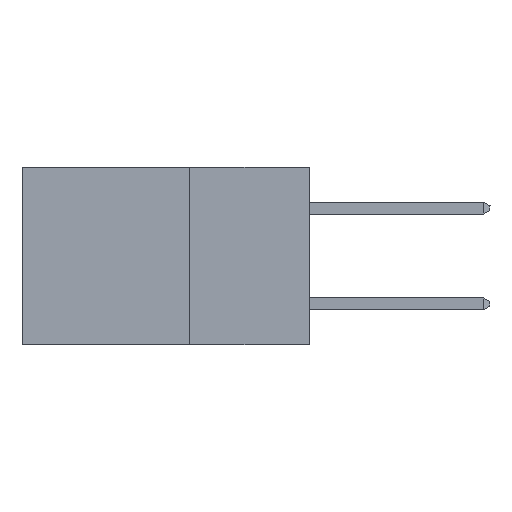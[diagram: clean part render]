
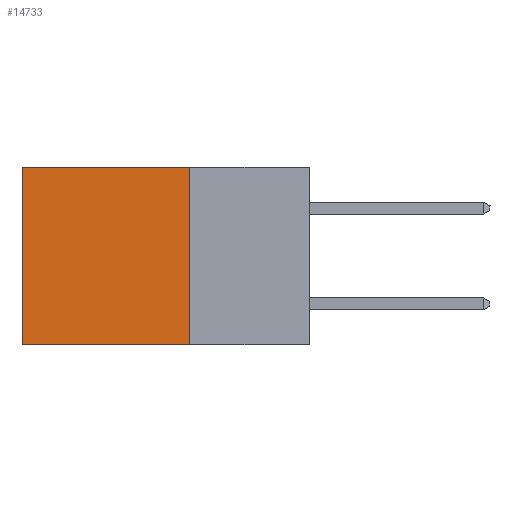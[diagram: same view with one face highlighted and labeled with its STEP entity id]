
A CAD part, left-side view. The second image highlights one B-rep face of the part: STEP entity #14733.
In plain terms, the highlighted planar face has unit normal (-1, 0, 0).
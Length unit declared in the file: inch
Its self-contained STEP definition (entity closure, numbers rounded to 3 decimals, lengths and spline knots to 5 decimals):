
#178 = VERTEX_POINT ( 'NONE', #4633 ) ;
#904 = LINE ( 'NONE', #6869, #1412 ) ;
#1408 = EDGE_CURVE ( 'NONE', #18609, #15009, #6712, .T. ) ;
#1412 = VECTOR ( 'NONE', #19752, 39.37008 ) ;
#1736 = CARTESIAN_POINT ( 'NONE',  ( 0.2875, 0.25, 0. ) ) ;
#2246 = CARTESIAN_POINT ( 'NONE',  ( 0.2875, 0.25, 0. ) ) ;
#3978 = AXIS2_PLACEMENT_3D ( 'NONE', #2246, #10109, #10245 ) ;
#4448 = ORIENTED_EDGE ( 'NONE', *, *, #20203, .F. ) ;
#4633 = CARTESIAN_POINT ( 'NONE',  ( 0.2875, 0.6, -0.37 ) ) ;
#5045 = LINE ( 'NONE', #8827, #16134 ) ;
#6611 = EDGE_LOOP ( 'NONE', ( #20382, #4448, #14657, #16684 ) ) ;
#6712 = LINE ( 'NONE', #8810, #16076 ) ;
#6869 = CARTESIAN_POINT ( 'NONE',  ( 0.2875, 0.6, 0. ) ) ;
#7322 = DIRECTION ( 'NONE',  ( 0., 1., 0. ) ) ;
#7566 = CARTESIAN_POINT ( 'NONE',  ( 0.2875, 0.25, -0.37 ) ) ;
#8810 = CARTESIAN_POINT ( 'NONE',  ( 0.2875, 0.25, 0. ) ) ;
#8827 = CARTESIAN_POINT ( 'NONE',  ( 0.2875, 0.25, -0.37 ) ) ;
#8958 = FACE_OUTER_BOUND ( 'NONE', #6611, .T. ) ;
#9757 = PLANE ( 'NONE',  #3978 ) ;
#10109 = DIRECTION ( 'NONE',  ( 1., 0., 0. ) ) ;
#10245 = DIRECTION ( 'NONE',  ( 0., 0., -1. ) ) ;
#11082 = LINE ( 'NONE', #18210, #13046 ) ;
#11723 = VERTEX_POINT ( 'NONE', #15837 ) ;
#13046 = VECTOR ( 'NONE', #19690, 39.37008 ) ;
#14657 = ORIENTED_EDGE ( 'NONE', *, *, #1408, .F. ) ;
#14733 = ADVANCED_FACE ( 'NONE', ( #8958 ), #9757, .F. ) ;
#15009 = VERTEX_POINT ( 'NONE', #7566 ) ;
#15837 = CARTESIAN_POINT ( 'NONE',  ( 0.2875, 0.6, 0. ) ) ;
#16076 = VECTOR ( 'NONE', #20045, 39.37008 ) ;
#16134 = VECTOR ( 'NONE', #7322, 39.37008 ) ;
#16684 = ORIENTED_EDGE ( 'NONE', *, *, #16767, .T. ) ;
#16767 = EDGE_CURVE ( 'NONE', #18609, #11723, #11082, .T. ) ;
#17724 = EDGE_CURVE ( 'NONE', #11723, #178, #904, .T. ) ;
#18210 = CARTESIAN_POINT ( 'NONE',  ( 0.2875, 0.25, 0. ) ) ;
#18609 = VERTEX_POINT ( 'NONE', #1736 ) ;
#19690 = DIRECTION ( 'NONE',  ( 0., 1., 0. ) ) ;
#19752 = DIRECTION ( 'NONE',  ( 0., 0., -1. ) ) ;
#20045 = DIRECTION ( 'NONE',  ( 0., 0., -1. ) ) ;
#20203 = EDGE_CURVE ( 'NONE', #15009, #178, #5045, .T. ) ;
#20382 = ORIENTED_EDGE ( 'NONE', *, *, #17724, .T. ) ;
